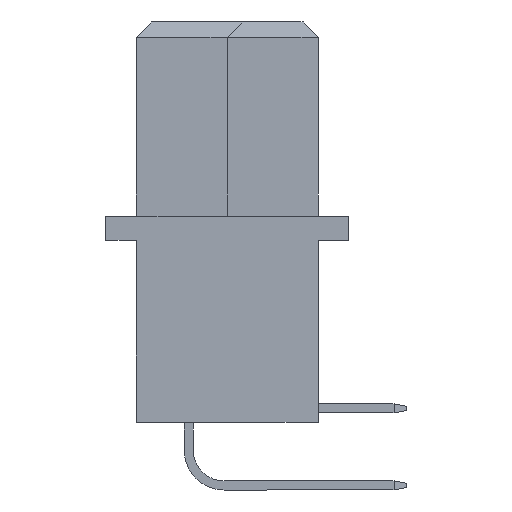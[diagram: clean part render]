
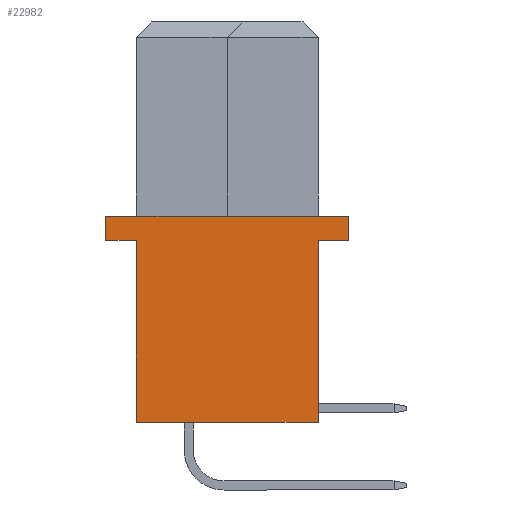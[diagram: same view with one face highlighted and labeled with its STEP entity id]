
A CAD part, left-side view. The second image highlights one B-rep face of the part: STEP entity #22982.
In plain terms, the highlighted planar face has unit normal (-1, 0, 0).
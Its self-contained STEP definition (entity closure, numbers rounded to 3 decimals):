
#2547 = VECTOR ( 'NONE', #27106, 1000. ) ;
#2642 = ORIENTED_EDGE ( 'NONE', *, *, #4177, .F. ) ;
#2679 = VERTEX_POINT ( 'NONE', #20891 ) ;
#2710 = VECTOR ( 'NONE', #18338, 1000. ) ;
#2767 = LINE ( 'NONE', #11320, #6937 ) ;
#3986 = CARTESIAN_POINT ( 'NONE',  ( -47., 4., -7.2 ) ) ;
#4149 = DIRECTION ( 'NONE',  ( 0., 0., 1. ) ) ;
#4177 = EDGE_CURVE ( 'NONE', #15215, #6276, #6047, .T. ) ;
#4660 = VERTEX_POINT ( 'NONE', #18712 ) ;
#5048 = VERTEX_POINT ( 'NONE', #10365 ) ;
#5119 = ORIENTED_EDGE ( 'NONE', *, *, #18173, .F. ) ;
#5216 = LINE ( 'NONE', #11771, #2710 ) ;
#5307 = ORIENTED_EDGE ( 'NONE', *, *, #7198, .F. ) ;
#5576 = ORIENTED_EDGE ( 'NONE', *, *, #22059, .F. ) ;
#6047 = LINE ( 'NONE', #14598, #12833 ) ;
#6165 = CARTESIAN_POINT ( 'NONE',  ( -47., -3., -7.2 ) ) ;
#6276 = VERTEX_POINT ( 'NONE', #3986 ) ;
#6401 = CARTESIAN_POINT ( 'NONE',  ( -47., -4., -6.4 ) ) ;
#6461 = LINE ( 'NONE', #11026, #13689 ) ;
#6937 = VECTOR ( 'NONE', #17615, 1000. ) ;
#7198 = EDGE_CURVE ( 'NONE', #16684, #4660, #10439, .T. ) ;
#7907 = EDGE_LOOP ( 'NONE', ( #5307, #5576, #15259, #27030, #5119, #2642, #12414, #26597 ) ) ;
#8434 = PLANE ( 'NONE',  #19058 ) ;
#9471 = EDGE_CURVE ( 'NONE', #2679, #4660, #14251, .T. ) ;
#10365 = CARTESIAN_POINT ( 'NONE',  ( -47., 4., -6.4 ) ) ;
#10439 = LINE ( 'NONE', #6165, #14101 ) ;
#10922 = CARTESIAN_POINT ( 'NONE',  ( -47., -3., -7.2 ) ) ;
#11026 = CARTESIAN_POINT ( 'NONE',  ( -47., -4., -13.2 ) ) ;
#11072 = DIRECTION ( 'NONE',  ( 0., 1., 0. ) ) ;
#11320 = CARTESIAN_POINT ( 'NONE',  ( -47., 3., -7.2 ) ) ;
#11771 = CARTESIAN_POINT ( 'NONE',  ( -47., 4., -6.4 ) ) ;
#11997 = CARTESIAN_POINT ( 'NONE',  ( -47., 4., -13.2 ) ) ;
#12414 = ORIENTED_EDGE ( 'NONE', *, *, #12474, .T. ) ;
#12474 = EDGE_CURVE ( 'NONE', #15215, #2679, #2767, .T. ) ;
#12833 = VECTOR ( 'NONE', #20888, 1000. ) ;
#12846 = CARTESIAN_POINT ( 'NONE',  ( -47., -4., -13.2 ) ) ;
#13157 = VERTEX_POINT ( 'NONE', #21378 ) ;
#13349 = LINE ( 'NONE', #10922, #17228 ) ;
#13689 = VECTOR ( 'NONE', #15159, 1000. ) ;
#14062 = CARTESIAN_POINT ( 'NONE',  ( -47., 3., -7.2 ) ) ;
#14101 = VECTOR ( 'NONE', #23269, 1000. ) ;
#14251 = LINE ( 'NONE', #20260, #14637 ) ;
#14598 = CARTESIAN_POINT ( 'NONE',  ( -47., 4., -7.2 ) ) ;
#14637 = VECTOR ( 'NONE', #22952, 1000. ) ;
#14978 = DIRECTION ( 'NONE',  ( -1., 0., 0. ) ) ;
#15159 = DIRECTION ( 'NONE',  ( 0., 0., 1. ) ) ;
#15215 = VERTEX_POINT ( 'NONE', #14062 ) ;
#15259 = ORIENTED_EDGE ( 'NONE', *, *, #25207, .T. ) ;
#16684 = VERTEX_POINT ( 'NONE', #17705 ) ;
#17228 = VECTOR ( 'NONE', #11072, 1000. ) ;
#17615 = DIRECTION ( 'NONE',  ( 0., 0., -1. ) ) ;
#17705 = CARTESIAN_POINT ( 'NONE',  ( -47., -3., -7.2 ) ) ;
#18173 = EDGE_CURVE ( 'NONE', #6276, #5048, #20697, .T. ) ;
#18338 = DIRECTION ( 'NONE',  ( 0., -1., 0. ) ) ;
#18379 = VERTEX_POINT ( 'NONE', #6401 ) ;
#18712 = CARTESIAN_POINT ( 'NONE',  ( -47., -3., -13.2 ) ) ;
#19058 = AXIS2_PLACEMENT_3D ( 'NONE', #12846, #14978, #4149 ) ;
#20260 = CARTESIAN_POINT ( 'NONE',  ( -47., -4., -13.2 ) ) ;
#20697 = LINE ( 'NONE', #11997, #2547 ) ;
#20888 = DIRECTION ( 'NONE',  ( 0., 1., 0. ) ) ;
#20891 = CARTESIAN_POINT ( 'NONE',  ( -47., 3., -13.2 ) ) ;
#21378 = CARTESIAN_POINT ( 'NONE',  ( -47., -4., -7.2 ) ) ;
#22059 = EDGE_CURVE ( 'NONE', #13157, #16684, #13349, .T. ) ;
#22952 = DIRECTION ( 'NONE',  ( 0., -1., 0. ) ) ;
#22982 = ADVANCED_FACE ( 'NONE', ( #27963 ), #8434, .T. ) ;
#23269 = DIRECTION ( 'NONE',  ( 0., 0., -1. ) ) ;
#23449 = EDGE_CURVE ( 'NONE', #5048, #18379, #5216, .T. ) ;
#25207 = EDGE_CURVE ( 'NONE', #13157, #18379, #6461, .T. ) ;
#26597 = ORIENTED_EDGE ( 'NONE', *, *, #9471, .T. ) ;
#27030 = ORIENTED_EDGE ( 'NONE', *, *, #23449, .F. ) ;
#27106 = DIRECTION ( 'NONE',  ( 0., 0., 1. ) ) ;
#27963 = FACE_OUTER_BOUND ( 'NONE', #7907, .T. ) ;
